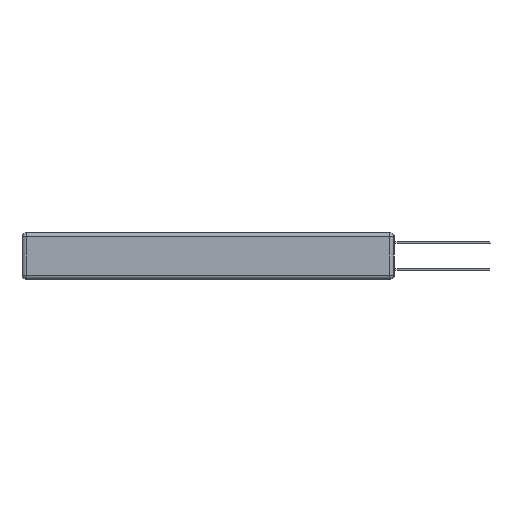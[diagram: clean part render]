
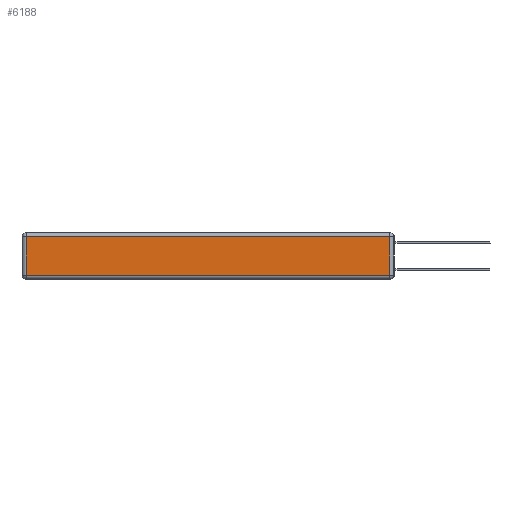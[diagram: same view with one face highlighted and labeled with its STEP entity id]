
A CAD part, left-side view. The second image highlights one B-rep face of the part: STEP entity #6188.
In plain terms, the highlighted planar face has unit normal (-1, 0, 0).
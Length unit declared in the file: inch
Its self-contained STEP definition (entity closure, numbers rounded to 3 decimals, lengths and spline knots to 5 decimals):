
#109 = VECTOR ( 'NONE', #9821, 39.37008 ) ;
#124 = CARTESIAN_POINT ( 'NONE',  ( 0., 2.72, -0.343 ) ) ;
#1543 = ORIENTED_EDGE ( 'NONE', *, *, #2386, .T. ) ;
#2386 = EDGE_CURVE ( 'NONE', #10437, #10955, #9826, .T. ) ;
#2685 = EDGE_CURVE ( 'NONE', #10863, #10437, #4248, .T. ) ;
#2802 = CARTESIAN_POINT ( 'NONE',  ( 0., 2.75, -0.03 ) ) ;
#3003 = DIRECTION ( 'NONE',  ( 0., 0., 1. ) ) ;
#3149 = CARTESIAN_POINT ( 'NONE',  ( 0., 0., -0.313 ) ) ;
#3242 = CARTESIAN_POINT ( 'NONE',  ( 0., 0.03, -0.313 ) ) ;
#3466 = CARTESIAN_POINT ( 'NONE',  ( 0., 2.72, -0.03 ) ) ;
#3729 = FACE_OUTER_BOUND ( 'NONE', #4135, .T. ) ;
#3883 = LINE ( 'NONE', #3149, #11892 ) ;
#3920 = CARTESIAN_POINT ( 'NONE',  ( 0., 2.72, -0.313 ) ) ;
#4135 = EDGE_LOOP ( 'NONE', ( #7090, #7157, #1543, #12432 ) ) ;
#4248 = LINE ( 'NONE', #9753, #9680 ) ;
#4951 = PLANE ( 'NONE',  #9175 ) ;
#5375 = EDGE_CURVE ( 'NONE', #10955, #6125, #5571, .T. ) ;
#5571 = LINE ( 'NONE', #124, #109 ) ;
#5919 = DIRECTION ( 'NONE',  ( -1., 0., 0. ) ) ;
#6097 = EDGE_CURVE ( 'NONE', #6125, #10863, #3883, .T. ) ;
#6125 = VERTEX_POINT ( 'NONE', #3920 ) ;
#6188 = ADVANCED_FACE ( 'NONE', ( #3729 ), #4951, .T. ) ;
#6363 = DIRECTION ( 'NONE',  ( 0., -1., 0. ) ) ;
#6536 = VECTOR ( 'NONE', #7711, 39.37008 ) ;
#6905 = DIRECTION ( 'NONE',  ( 0., 0., 1. ) ) ;
#7090 = ORIENTED_EDGE ( 'NONE', *, *, #6097, .T. ) ;
#7157 = ORIENTED_EDGE ( 'NONE', *, *, #2685, .T. ) ;
#7711 = DIRECTION ( 'NONE',  ( 0., 1., 0. ) ) ;
#9175 = AXIS2_PLACEMENT_3D ( 'NONE', #10719, #5919, #3003 ) ;
#9680 = VECTOR ( 'NONE', #6905, 39.37008 ) ;
#9753 = CARTESIAN_POINT ( 'NONE',  ( 0., 0.03, -0.343 ) ) ;
#9821 = DIRECTION ( 'NONE',  ( 0., 0., -1. ) ) ;
#9826 = LINE ( 'NONE', #2802, #6536 ) ;
#10437 = VERTEX_POINT ( 'NONE', #11345 ) ;
#10719 = CARTESIAN_POINT ( 'NONE',  ( 0., 0., -0.343 ) ) ;
#10863 = VERTEX_POINT ( 'NONE', #3242 ) ;
#10955 = VERTEX_POINT ( 'NONE', #3466 ) ;
#11345 = CARTESIAN_POINT ( 'NONE',  ( 0., 0.03, -0.03 ) ) ;
#11892 = VECTOR ( 'NONE', #6363, 39.37008 ) ;
#12432 = ORIENTED_EDGE ( 'NONE', *, *, #5375, .T. ) ;
